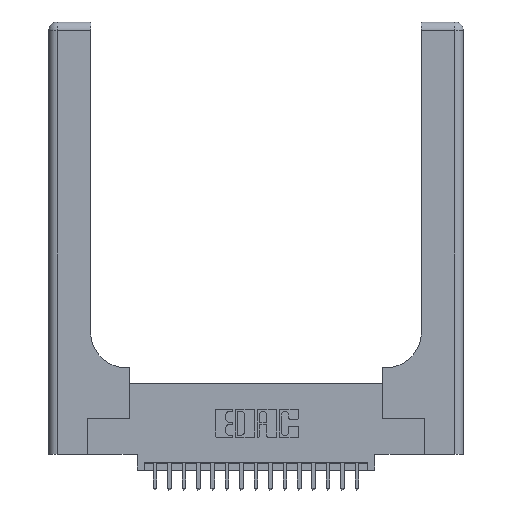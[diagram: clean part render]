
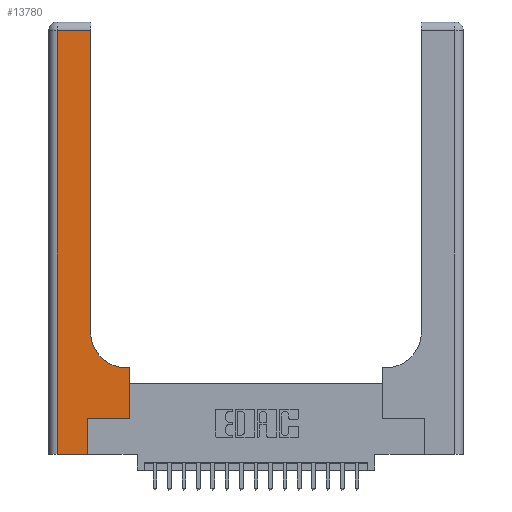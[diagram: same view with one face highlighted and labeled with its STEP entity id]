
A CAD part, top view. The second image highlights one B-rep face of the part: STEP entity #13780.
In plain terms, the highlighted planar face has unit normal (0, 0, 1).
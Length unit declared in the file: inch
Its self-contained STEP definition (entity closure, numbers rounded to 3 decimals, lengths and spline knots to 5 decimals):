
#18 = DIRECTION ( 'NONE',  ( -1., 0., 0. ) ) ;
#467 = ORIENTED_EDGE ( 'NONE', *, *, #4374, .T. ) ;
#1201 = VERTEX_POINT ( 'NONE', #6195 ) ;
#1311 = CARTESIAN_POINT ( 'NONE',  ( 0.2915, 0.6, 0.37 ) ) ;
#2691 = LINE ( 'NONE', #18451, #16675 ) ;
#3004 = EDGE_LOOP ( 'NONE', ( #6605, #10211, #6976, #16152, #15513, #467, #18407, #11916, #3669 ) ) ;
#3099 = CARTESIAN_POINT ( 'NONE',  ( 0.269, 0., 0.37 ) ) ;
#3120 = CARTESIAN_POINT ( 'NONE',  ( 0.06, 3., 0.37 ) ) ;
#3199 = PLANE ( 'NONE',  #7667 ) ;
#3261 = EDGE_CURVE ( 'NONE', #1201, #17715, #9029, .T. ) ;
#3546 = VERTEX_POINT ( 'NONE', #14798 ) ;
#3646 = CARTESIAN_POINT ( 'NONE',  ( 0.5585, 0.25, 0.37 ) ) ;
#3669 = ORIENTED_EDGE ( 'NONE', *, *, #18796, .T. ) ;
#3921 = CARTESIAN_POINT ( 'NONE',  ( 0.5585, 0.25, 0.37 ) ) ;
#4259 = CARTESIAN_POINT ( 'NONE',  ( 0., 0., 0.37 ) ) ;
#4374 = EDGE_CURVE ( 'NONE', #10599, #19861, #2691, .T. ) ;
#5453 = EDGE_CURVE ( 'NONE', #19861, #3546, #20228, .T. ) ;
#5596 = DIRECTION ( 'NONE',  ( 1., 0., 0. ) ) ;
#6195 = CARTESIAN_POINT ( 'NONE',  ( 0.06, 0., 0.37 ) ) ;
#6260 = VECTOR ( 'NONE', #12669, 39.37008 ) ;
#6377 = VECTOR ( 'NONE', #9249, 39.37008 ) ;
#6437 = DIRECTION ( 'NONE',  ( 0., 0., -1. ) ) ;
#6605 = ORIENTED_EDGE ( 'NONE', *, *, #19934, .T. ) ;
#6976 = ORIENTED_EDGE ( 'NONE', *, *, #17013, .T. ) ;
#7009 = CARTESIAN_POINT ( 'NONE',  ( 0.5415, 0.6, 0.37 ) ) ;
#7102 = CARTESIAN_POINT ( 'NONE',  ( 0.2915, 3., 0.37 ) ) ;
#7562 = VERTEX_POINT ( 'NONE', #16844 ) ;
#7667 = AXIS2_PLACEMENT_3D ( 'NONE', #12881, #6437, #14206 ) ;
#8261 = VECTOR ( 'NONE', #10312, 39.37008 ) ;
#8764 = CARTESIAN_POINT ( 'NONE',  ( 0.2915, 2.94, 0.37 ) ) ;
#8971 = DIRECTION ( 'NONE',  ( 1., 0., 0. ) ) ;
#9029 = LINE ( 'NONE', #4259, #13288 ) ;
#9134 = LINE ( 'NONE', #1311, #6377 ) ;
#9249 = DIRECTION ( 'NONE',  ( -1., 0., 0. ) ) ;
#9291 = LINE ( 'NONE', #14142, #16752 ) ;
#10030 = VERTEX_POINT ( 'NONE', #13848 ) ;
#10211 = ORIENTED_EDGE ( 'NONE', *, *, #13712, .T. ) ;
#10312 = DIRECTION ( 'NONE',  ( 0., 1., 0. ) ) ;
#10526 = AXIS2_PLACEMENT_3D ( 'NONE', #16549, #19780, #5596 ) ;
#10599 = VERTEX_POINT ( 'NONE', #12493 ) ;
#10707 = DIRECTION ( 'NONE',  ( 1., 0., 0. ) ) ;
#11041 = CARTESIAN_POINT ( 'NONE',  ( 0.269, 0., 0.37 ) ) ;
#11593 = EDGE_CURVE ( 'NONE', #3546, #11897, #9134, .T. ) ;
#11897 = VERTEX_POINT ( 'NONE', #7009 ) ;
#11916 = ORIENTED_EDGE ( 'NONE', *, *, #11593, .T. ) ;
#12493 = CARTESIAN_POINT ( 'NONE',  ( 0.269, 0.25, 0.37 ) ) ;
#12669 = DIRECTION ( 'NONE',  ( 0., 1., 0. ) ) ;
#12668 = DIRECTION ( 'NONE',  ( 0., -1., 0. ) ) ;
#12881 = CARTESIAN_POINT ( 'NONE',  ( 0., 3., 0.37 ) ) ;
#13288 = VECTOR ( 'NONE', #8971, 39.37008 ) ;
#13597 = VERTEX_POINT ( 'NONE', #8764 ) ;
#13712 = EDGE_CURVE ( 'NONE', #13597, #10030, #9291, .T. ) ;
#13780 = ADVANCED_FACE ( 'NONE', ( #16258 ), #3199, .F. ) ;
#13829 = EDGE_CURVE ( 'NONE', #17715, #10599, #14038, .T. ) ;
#13848 = CARTESIAN_POINT ( 'NONE',  ( 0.06, 2.94, 0.37 ) ) ;
#13866 = LINE ( 'NONE', #3120, #16080 ) ;
#14038 = LINE ( 'NONE', #11041, #6260 ) ;
#14142 = CARTESIAN_POINT ( 'NONE',  ( 0., 2.94, 0.37 ) ) ;
#14206 = DIRECTION ( 'NONE',  ( -1., 0., 0. ) ) ;
#14480 = VECTOR ( 'NONE', #18193, 39.37008 ) ;
#14798 = CARTESIAN_POINT ( 'NONE',  ( 0.5585, 0.6, 0.37 ) ) ;
#15007 = LINE ( 'NONE', #7102, #8261 ) ;
#15305 = CIRCLE ( 'NONE', #10526, 0.25 ) ;
#15513 = ORIENTED_EDGE ( 'NONE', *, *, #13829, .T. ) ;
#16080 = VECTOR ( 'NONE', #12668, 39.37008 ) ;
#16152 = ORIENTED_EDGE ( 'NONE', *, *, #3261, .T. ) ;
#16258 = FACE_OUTER_BOUND ( 'NONE', #3004, .T. ) ;
#16549 = CARTESIAN_POINT ( 'NONE',  ( 0.5415, 0.85, 0.37 ) ) ;
#16675 = VECTOR ( 'NONE', #10707, 39.37008 ) ;
#16752 = VECTOR ( 'NONE', #18, 39.37008 ) ;
#16844 = CARTESIAN_POINT ( 'NONE',  ( 0.2915, 0.85, 0.37 ) ) ;
#17013 = EDGE_CURVE ( 'NONE', #10030, #1201, #13866, .T. ) ;
#17715 = VERTEX_POINT ( 'NONE', #3099 ) ;
#18193 = DIRECTION ( 'NONE',  ( 0., 1., 0. ) ) ;
#18407 = ORIENTED_EDGE ( 'NONE', *, *, #5453, .T. ) ;
#18451 = CARTESIAN_POINT ( 'NONE',  ( 0.269, 0.25, 0.37 ) ) ;
#18796 = EDGE_CURVE ( 'NONE', #11897, #7562, #15305, .T. ) ;
#19780 = DIRECTION ( 'NONE',  ( 0., 0., -1. ) ) ;
#19861 = VERTEX_POINT ( 'NONE', #3646 ) ;
#19934 = EDGE_CURVE ( 'NONE', #7562, #13597, #15007, .T. ) ;
#20228 = LINE ( 'NONE', #3921, #14480 ) ;
